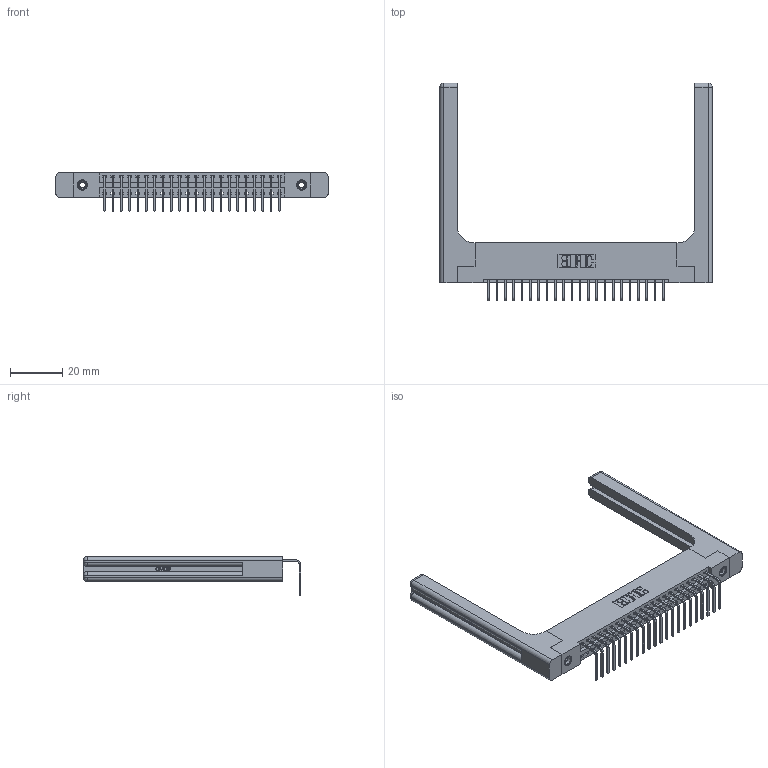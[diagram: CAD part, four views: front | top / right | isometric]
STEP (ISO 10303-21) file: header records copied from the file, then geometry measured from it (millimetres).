
FILE_DESCRIPTION (( 'STEP AP203' ), '1' );
FILE_NAME ('396-022-558-158.STEP', '2019-11-01T06:17:55', ( '' ), ( '' ), 'SwSTEP 2.0', 'SolidWorks 2016', '' );
FILE_SCHEMA (( 'CONFIG_CONTROL_DESIGN' ));
Length unit declared in the file: inch
Products named in the file (5): 346-220-058_345-220-058; 396-022-558-158; 346 Part_Flush Mounting Lugs - 0.156 Dia-TH; 345-292-001_558 Tail - 2; 345-250-001_345-250-001-102
Assembly tree (27 placements, depth 2):
  396-022-558-158
    346 Part_Flush Mounting Lugs - 0.156 Dia-TH
    345-292-001_558 Tail - 2  x22
    345-250-001_345-250-001-102  x2
    346-220-058_345-220-058  x2
Bounding box: 103.91 x 83.12 x 14.73 mm (x, y, z)
Volume: 17400.5 mm3; surface area: 17742.4 mm2
Topology: 27 solids, 27 shells, 1698 faces, 4999 edges, 3282 vertices
Faces by surface type: plane 1148, cylinder 490, bspline 36, cone 12, sphere 8, torus 4
Entity records: 21612 total; most frequent: CARTESIAN_POINT 4691, ORIENTED_EDGE 3444, DIRECTION 3094, EDGE_CURVE 1722, LINE 1410, VECTOR 1410, VERTEX_POINT 1138, AXIS2_PLACEMENT_3D 842
